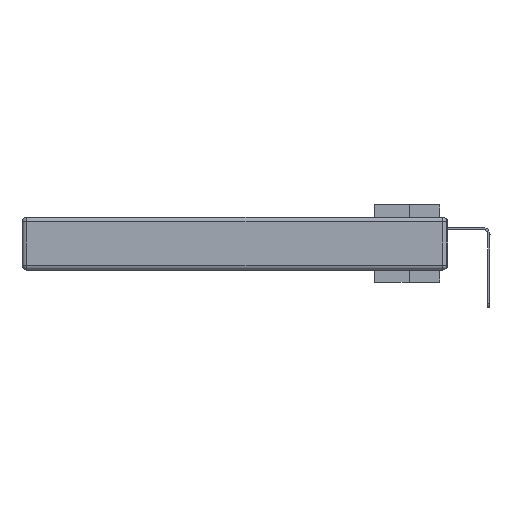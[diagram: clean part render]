
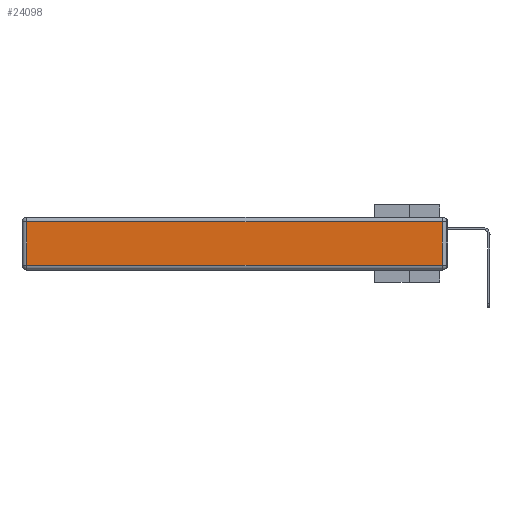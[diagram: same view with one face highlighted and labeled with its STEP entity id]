
A CAD part, left-side view. The second image highlights one B-rep face of the part: STEP entity #24098.
In plain terms, the highlighted planar face has unit normal (-1, 0, 0).
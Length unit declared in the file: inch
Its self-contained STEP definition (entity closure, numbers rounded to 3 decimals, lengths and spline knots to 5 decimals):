
#224 = VECTOR ( 'NONE', #16061, 39.37008 ) ;
#796 = LINE ( 'NONE', #2629, #3163 ) ;
#1829 = ORIENTED_EDGE ( 'NONE', *, *, #6504, .T. ) ;
#2121 = LINE ( 'NONE', #3136, #6428 ) ;
#2142 = EDGE_CURVE ( 'NONE', #30636, #13709, #2121, .T. ) ;
#2629 = CARTESIAN_POINT ( 'NONE',  ( 0., 0., -0.313 ) ) ;
#3136 = CARTESIAN_POINT ( 'NONE',  ( 0., 2.72, -0.343 ) ) ;
#3163 = VECTOR ( 'NONE', #4695, 39.37008 ) ;
#3916 = EDGE_CURVE ( 'NONE', #13709, #8379, #796, .T. ) ;
#4695 = DIRECTION ( 'NONE',  ( 0., -1., 0. ) ) ;
#6080 = FACE_OUTER_BOUND ( 'NONE', #21438, .T. ) ;
#6149 = VECTOR ( 'NONE', #15875, 39.37008 ) ;
#6428 = VECTOR ( 'NONE', #25577, 39.37008 ) ;
#6504 = EDGE_CURVE ( 'NONE', #30114, #30636, #6908, .T. ) ;
#6908 = LINE ( 'NONE', #8453, #224 ) ;
#6935 = LINE ( 'NONE', #30417, #6149 ) ;
#8379 = VERTEX_POINT ( 'NONE', #30131 ) ;
#8453 = CARTESIAN_POINT ( 'NONE',  ( 0., 2.75, -0.03 ) ) ;
#11420 = ORIENTED_EDGE ( 'NONE', *, *, #2142, .T. ) ;
#13220 = AXIS2_PLACEMENT_3D ( 'NONE', #28254, #21054, #23478 ) ;
#13709 = VERTEX_POINT ( 'NONE', #22528 ) ;
#15399 = CARTESIAN_POINT ( 'NONE',  ( 0., 2.72, -0.03 ) ) ;
#15875 = DIRECTION ( 'NONE',  ( 0., 0., 1. ) ) ;
#16061 = DIRECTION ( 'NONE',  ( 0., 1., 0. ) ) ;
#18680 = ORIENTED_EDGE ( 'NONE', *, *, #19188, .T. ) ;
#19188 = EDGE_CURVE ( 'NONE', #8379, #30114, #6935, .T. ) ;
#21054 = DIRECTION ( 'NONE',  ( -1., 0., 0. ) ) ;
#21438 = EDGE_LOOP ( 'NONE', ( #28804, #18680, #1829, #11420 ) ) ;
#22528 = CARTESIAN_POINT ( 'NONE',  ( 0., 2.72, -0.313 ) ) ;
#23478 = DIRECTION ( 'NONE',  ( 0., 0., 1. ) ) ;
#24098 = ADVANCED_FACE ( 'NONE', ( #6080 ), #31123, .T. ) ;
#25577 = DIRECTION ( 'NONE',  ( 0., 0., -1. ) ) ;
#26916 = CARTESIAN_POINT ( 'NONE',  ( 0., 0.03, -0.03 ) ) ;
#28254 = CARTESIAN_POINT ( 'NONE',  ( 0., 0., -0.343 ) ) ;
#28804 = ORIENTED_EDGE ( 'NONE', *, *, #3916, .T. ) ;
#30114 = VERTEX_POINT ( 'NONE', #26916 ) ;
#30131 = CARTESIAN_POINT ( 'NONE',  ( 0., 0.03, -0.313 ) ) ;
#30417 = CARTESIAN_POINT ( 'NONE',  ( 0., 0.03, -0.343 ) ) ;
#30636 = VERTEX_POINT ( 'NONE', #15399 ) ;
#31123 = PLANE ( 'NONE',  #13220 ) ;
